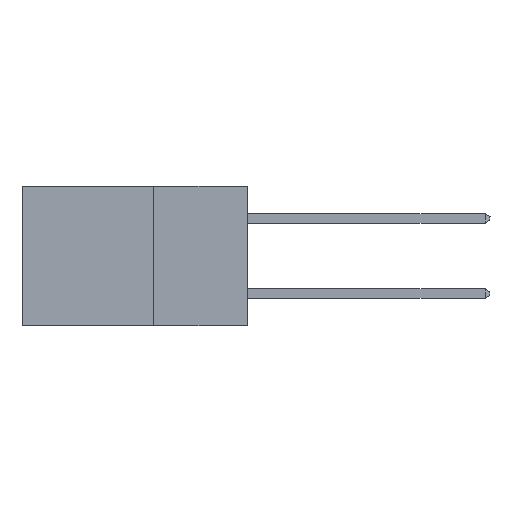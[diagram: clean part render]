
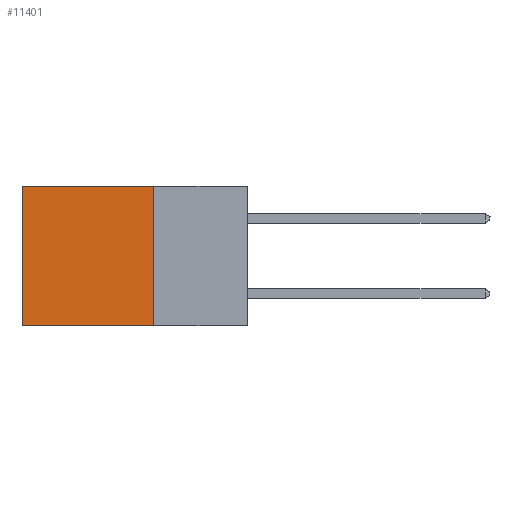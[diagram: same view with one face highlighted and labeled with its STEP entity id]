
A CAD part, left-side view. The second image highlights one B-rep face of the part: STEP entity #11401.
In plain terms, the highlighted planar face has unit normal (-1, 0, 0).
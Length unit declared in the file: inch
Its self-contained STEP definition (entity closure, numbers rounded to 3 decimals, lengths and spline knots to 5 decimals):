
#133 = LINE ( 'NONE', #6738, #11425 ) ;
#1906 = CARTESIAN_POINT ( 'NONE',  ( 0.298, 0.25, -0.37 ) ) ;
#2650 = VECTOR ( 'NONE', #11114, 39.37008 ) ;
#3169 = DIRECTION ( 'NONE',  ( 1., 0., 0. ) ) ;
#3321 = DIRECTION ( 'NONE',  ( 0., 0., -1. ) ) ;
#4838 = DIRECTION ( 'NONE',  ( 0., 0., -1. ) ) ;
#5313 = VECTOR ( 'NONE', #15665, 39.37008 ) ;
#5648 = LINE ( 'NONE', #22723, #19464 ) ;
#6738 = CARTESIAN_POINT ( 'NONE',  ( 0.298, 0.6, 0. ) ) ;
#7168 = VERTEX_POINT ( 'NONE', #13531 ) ;
#7640 = ORIENTED_EDGE ( 'NONE', *, *, #10877, .F. ) ;
#8461 = DIRECTION ( 'NONE',  ( 0., 0., -1. ) ) ;
#9143 = CARTESIAN_POINT ( 'NONE',  ( 0.298, 0.25, -0.37 ) ) ;
#10109 = VERTEX_POINT ( 'NONE', #20270 ) ;
#10877 = EDGE_CURVE ( 'NONE', #7168, #16197, #5648, .T. ) ;
#11114 = DIRECTION ( 'NONE',  ( 0., 1., 0. ) ) ;
#11197 = ORIENTED_EDGE ( 'NONE', *, *, #18650, .F. ) ;
#11401 = ADVANCED_FACE ( 'NONE', ( #16247 ), #19660, .F. ) ;
#11425 = VECTOR ( 'NONE', #4838, 39.37008 ) ;
#13183 = ORIENTED_EDGE ( 'NONE', *, *, #13880, .T. ) ;
#13531 = CARTESIAN_POINT ( 'NONE',  ( 0.298, 0.25, 0. ) ) ;
#13880 = EDGE_CURVE ( 'NONE', #7168, #10109, #15162, .T. ) ;
#13957 = CARTESIAN_POINT ( 'NONE',  ( 0.298, 0.25, 0. ) ) ;
#15162 = LINE ( 'NONE', #23156, #5313 ) ;
#15354 = ORIENTED_EDGE ( 'NONE', *, *, #18059, .T. ) ;
#15665 = DIRECTION ( 'NONE',  ( 0., 1., 0. ) ) ;
#15912 = LINE ( 'NONE', #9143, #2650 ) ;
#16197 = VERTEX_POINT ( 'NONE', #1906 ) ;
#16247 = FACE_OUTER_BOUND ( 'NONE', #16539, .T. ) ;
#16539 = EDGE_LOOP ( 'NONE', ( #15354, #11197, #7640, #13183 ) ) ;
#17289 = AXIS2_PLACEMENT_3D ( 'NONE', #13957, #3169, #3321 ) ;
#18059 = EDGE_CURVE ( 'NONE', #10109, #23426, #133, .T. ) ;
#18650 = EDGE_CURVE ( 'NONE', #16197, #23426, #15912, .T. ) ;
#19464 = VECTOR ( 'NONE', #8461, 39.37008 ) ;
#19660 = PLANE ( 'NONE',  #17289 ) ;
#20270 = CARTESIAN_POINT ( 'NONE',  ( 0.298, 0.6, 0. ) ) ;
#21787 = CARTESIAN_POINT ( 'NONE',  ( 0.298, 0.6, -0.37 ) ) ;
#22723 = CARTESIAN_POINT ( 'NONE',  ( 0.298, 0.25, 0. ) ) ;
#23156 = CARTESIAN_POINT ( 'NONE',  ( 0.298, 0.25, 0. ) ) ;
#23426 = VERTEX_POINT ( 'NONE', #21787 ) ;
